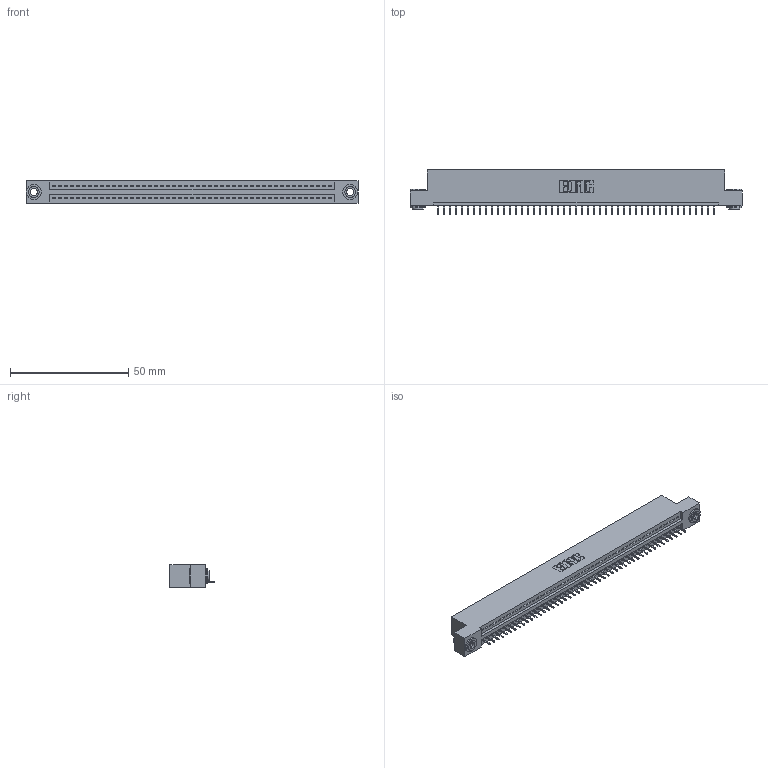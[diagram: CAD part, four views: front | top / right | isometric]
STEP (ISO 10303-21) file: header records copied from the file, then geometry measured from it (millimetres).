
FILE_DESCRIPTION (( 'STEP AP203' ), '1' );
FILE_NAME ('895-047-525-103.STEP', '2020-09-27T06:11:53', ( '' ), ( '' ), 'SwSTEP 2.0', 'SolidWorks 2020', '' );
FILE_SCHEMA (( 'CONFIG_CONTROL_DESIGN' ));
Length unit declared in the file: inch
Products named in the file (4): 895-047-525-103; 345-292-001_345-293-125; 345-250-002_345-250-002-102; 845 Part_Flush Mounting Lugs - 0.156 Dia-TH
Assembly tree (50 placements, depth 2):
  895-047-525-103
    845 Part_Flush Mounting Lugs - 0.156 Dia-TH
    345-292-001_345-293-125  x47
    345-250-002_345-250-002-102  x2
Bounding box: 140.59 x 18.72 x 9.4 mm (x, y, z)
Volume: 13221.7 mm3; surface area: 17213 mm2
Topology: 50 solids, 50 shells, 3078 faces, 8877 edges, 5726 vertices
Faces by surface type: plane 2252, cylinder 818, cone 8
Entity records: 35424 total; most frequent: CARTESIAN_POINT 6112, ORIENTED_EDGE 6086, DIRECTION 5363, EDGE_CURVE 3043, LINE 2703, VECTOR 2703, VERTEX_POINT 2022, AXIS2_PLACEMENT_3D 1330
